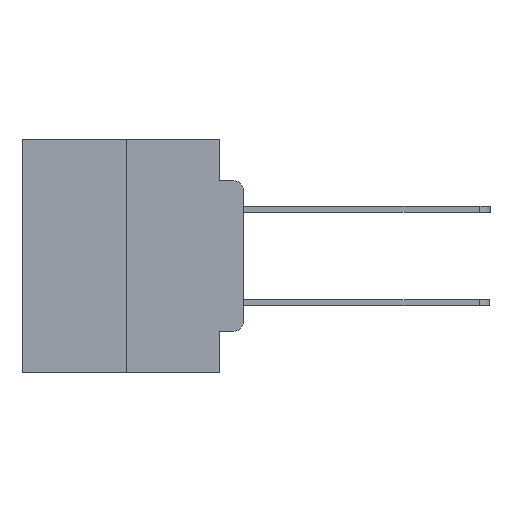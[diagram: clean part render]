
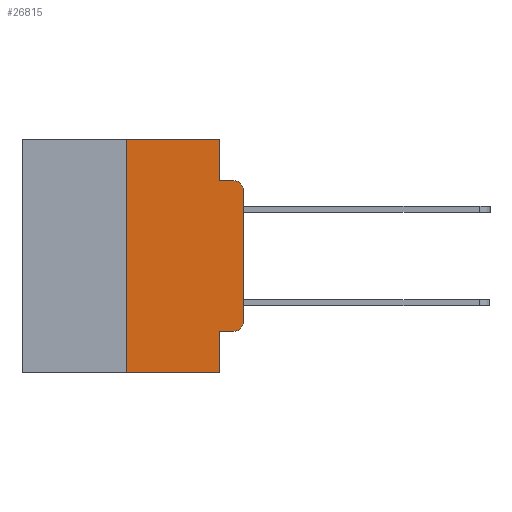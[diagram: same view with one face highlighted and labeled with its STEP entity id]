
A CAD part, left-side view. The second image highlights one B-rep face of the part: STEP entity #26815.
In plain terms, the highlighted planar face has unit normal (-1, 0, 0).
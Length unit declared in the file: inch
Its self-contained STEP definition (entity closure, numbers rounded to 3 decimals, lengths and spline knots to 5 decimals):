
#372 = VERTEX_POINT ( 'NONE', #26856 ) ;
#595 = CARTESIAN_POINT ( 'NONE',  ( 0., 0.02, -0.3915 ) ) ;
#979 = DIRECTION ( 'NONE',  ( 0., 0., -1. ) ) ;
#1356 = VECTOR ( 'NONE', #8922, 39.37008 ) ;
#2092 = LINE ( 'NONE', #4792, #9163 ) ;
#2120 = CARTESIAN_POINT ( 'NONE',  ( 0., 0.051, 0. ) ) ;
#2789 = LINE ( 'NONE', #6039, #19749 ) ;
#2810 = DIRECTION ( 'NONE',  ( 0., 0., -1. ) ) ;
#3122 = CARTESIAN_POINT ( 'NONE',  ( 0., 0., -0.3915 ) ) ;
#3253 = ORIENTED_EDGE ( 'NONE', *, *, #15903, .T. ) ;
#3830 = DIRECTION ( 'NONE',  ( 0., 0., -1. ) ) ;
#3937 = ORIENTED_EDGE ( 'NONE', *, *, #18745, .F. ) ;
#4391 = VECTOR ( 'NONE', #6496, 39.37008 ) ;
#4705 = EDGE_LOOP ( 'NONE', ( #3253, #8956, #3937, #9612, #10285, #15905, #17223, #7270, #13608, #19204 ) ) ;
#4792 = CARTESIAN_POINT ( 'NONE',  ( 0., 0., 0. ) ) ;
#4942 = VERTEX_POINT ( 'NONE', #23780 ) ;
#5264 = AXIS2_PLACEMENT_3D ( 'NONE', #8042, #16554, #3830 ) ;
#5629 = CARTESIAN_POINT ( 'NONE',  ( 0., 0.051, 0. ) ) ;
#6039 = CARTESIAN_POINT ( 'NONE',  ( 0., 0.051, -0.0885 ) ) ;
#6329 = VERTEX_POINT ( 'NONE', #11685 ) ;
#6419 = LINE ( 'NONE', #15217, #1356 ) ;
#6496 = DIRECTION ( 'NONE',  ( 0., -1., 0. ) ) ;
#6893 = VECTOR ( 'NONE', #18048, 39.37008 ) ;
#6958 = DIRECTION ( 'NONE',  ( 0., 0., 1. ) ) ;
#7270 = ORIENTED_EDGE ( 'NONE', *, *, #18206, .F. ) ;
#7870 = CARTESIAN_POINT ( 'NONE',  ( 0., 0.051, 0. ) ) ;
#8042 = CARTESIAN_POINT ( 'NONE',  ( 0., 0.473, 0. ) ) ;
#8721 = VERTEX_POINT ( 'NONE', #7870 ) ;
#8922 = DIRECTION ( 'NONE',  ( 0., -1., 0. ) ) ;
#8956 = ORIENTED_EDGE ( 'NONE', *, *, #13085, .T. ) ;
#9163 = VECTOR ( 'NONE', #6958, 39.37008 ) ;
#9612 = ORIENTED_EDGE ( 'NONE', *, *, #17312, .F. ) ;
#9628 = CARTESIAN_POINT ( 'NONE',  ( 0., 0.25, 0. ) ) ;
#10285 = ORIENTED_EDGE ( 'NONE', *, *, #20834, .F. ) ;
#10756 = LINE ( 'NONE', #10803, #4391 ) ;
#10803 = CARTESIAN_POINT ( 'NONE',  ( 0., 0.473, 0. ) ) ;
#11123 = EDGE_CURVE ( 'NONE', #4942, #19139, #18093, .T. ) ;
#11685 = CARTESIAN_POINT ( 'NONE',  ( 0., 0.25, 0. ) ) ;
#13085 = EDGE_CURVE ( 'NONE', #21315, #24309, #21864, .T. ) ;
#13230 = LINE ( 'NONE', #9628, #6893 ) ;
#13502 = CARTESIAN_POINT ( 'NONE',  ( 0., 0.02, -0.0885 ) ) ;
#13608 = ORIENTED_EDGE ( 'NONE', *, *, #19616, .T. ) ;
#13732 = VERTEX_POINT ( 'NONE', #20229 ) ;
#13824 = DIRECTION ( 'NONE',  ( -1., 0., 0. ) ) ;
#14058 = AXIS2_PLACEMENT_3D ( 'NONE', #26307, #13824, #979 ) ;
#14342 = DIRECTION ( 'NONE',  ( 0., -1., 0. ) ) ;
#14368 = CARTESIAN_POINT ( 'NONE',  ( 0., 0.25, -0.5 ) ) ;
#14445 = PLANE ( 'NONE',  #5264 ) ;
#14583 = CARTESIAN_POINT ( 'NONE',  ( 0., 0., -0.1085 ) ) ;
#15217 = CARTESIAN_POINT ( 'NONE',  ( 0., 0.051, -0.4115 ) ) ;
#15582 = DIRECTION ( 'NONE',  ( -1., 0., 0. ) ) ;
#15861 = CARTESIAN_POINT ( 'NONE',  ( 0., 0.051, -0.4115 ) ) ;
#15903 = EDGE_CURVE ( 'NONE', #19139, #21315, #2092, .T. ) ;
#15905 = ORIENTED_EDGE ( 'NONE', *, *, #23791, .F. ) ;
#16554 = DIRECTION ( 'NONE',  ( 1., 0., 0. ) ) ;
#16841 = EDGE_CURVE ( 'NONE', #21876, #372, #23895, .T. ) ;
#17200 = AXIS2_PLACEMENT_3D ( 'NONE', #595, #15582, #2810 ) ;
#17223 = ORIENTED_EDGE ( 'NONE', *, *, #16841, .T. ) ;
#17312 = EDGE_CURVE ( 'NONE', #8721, #13732, #17674, .T. ) ;
#17674 = LINE ( 'NONE', #5629, #23248 ) ;
#18048 = DIRECTION ( 'NONE',  ( 0., 0., 1. ) ) ;
#18093 = CIRCLE ( 'NONE', #17200, 0.02 ) ;
#18206 = EDGE_CURVE ( 'NONE', #25052, #372, #22550, .T. ) ;
#18373 = VECTOR ( 'NONE', #14342, 39.37008 ) ;
#18490 = CARTESIAN_POINT ( 'NONE',  ( 0., 0.473, -0.5 ) ) ;
#18745 = EDGE_CURVE ( 'NONE', #13732, #24309, #2789, .T. ) ;
#19139 = VERTEX_POINT ( 'NONE', #3122 ) ;
#19143 = DIRECTION ( 'NONE',  ( 0., 0., -1. ) ) ;
#19204 = ORIENTED_EDGE ( 'NONE', *, *, #11123, .T. ) ;
#19616 = EDGE_CURVE ( 'NONE', #25052, #4942, #6419, .T. ) ;
#19749 = VECTOR ( 'NONE', #20878, 39.37008 ) ;
#20229 = CARTESIAN_POINT ( 'NONE',  ( 0., 0.051, -0.0885 ) ) ;
#20834 = EDGE_CURVE ( 'NONE', #6329, #8721, #10756, .T. ) ;
#20878 = DIRECTION ( 'NONE',  ( 0., -1., 0. ) ) ;
#21315 = VERTEX_POINT ( 'NONE', #14583 ) ;
#21864 = CIRCLE ( 'NONE', #14058, 0.02 ) ;
#21876 = VERTEX_POINT ( 'NONE', #14368 ) ;
#22550 = LINE ( 'NONE', #2120, #23199 ) ;
#23199 = VECTOR ( 'NONE', #19143, 39.37008 ) ;
#23248 = VECTOR ( 'NONE', #26595, 39.37008 ) ;
#23780 = CARTESIAN_POINT ( 'NONE',  ( 0., 0.02, -0.4115 ) ) ;
#23791 = EDGE_CURVE ( 'NONE', #21876, #6329, #13230, .T. ) ;
#23895 = LINE ( 'NONE', #18490, #18373 ) ;
#24309 = VERTEX_POINT ( 'NONE', #13502 ) ;
#25052 = VERTEX_POINT ( 'NONE', #15861 ) ;
#26307 = CARTESIAN_POINT ( 'NONE',  ( 0., 0.02, -0.1085 ) ) ;
#26595 = DIRECTION ( 'NONE',  ( 0., 0., -1. ) ) ;
#26606 = FACE_OUTER_BOUND ( 'NONE', #4705, .T. ) ;
#26815 = ADVANCED_FACE ( 'NONE', ( #26606 ), #14445, .F. ) ;
#26856 = CARTESIAN_POINT ( 'NONE',  ( 0., 0.051, -0.5 ) ) ;
